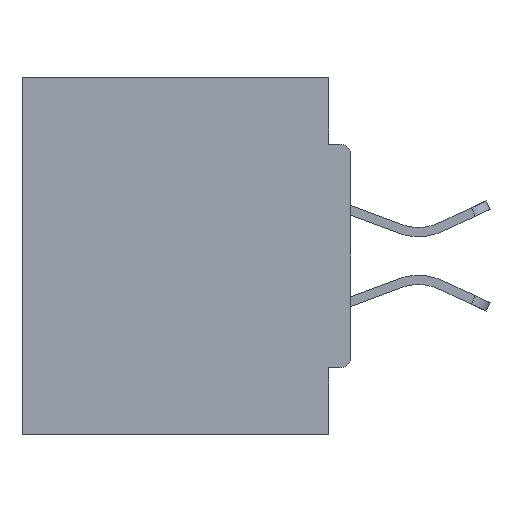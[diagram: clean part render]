
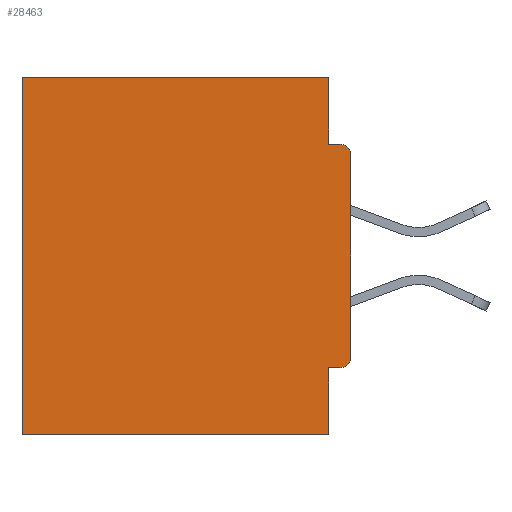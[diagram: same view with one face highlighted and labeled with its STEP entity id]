
A CAD part, left-side view. The second image highlights one B-rep face of the part: STEP entity #28463.
In plain terms, the highlighted planar face has unit normal (-1, 0, 0).
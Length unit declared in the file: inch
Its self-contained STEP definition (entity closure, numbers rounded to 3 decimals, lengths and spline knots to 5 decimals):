
#237 = CARTESIAN_POINT ( 'NONE',  ( 0.298, 0., -0.0935 ) ) ;
#345 = LINE ( 'NONE', #13694, #14508 ) ;
#370 = CARTESIAN_POINT ( 'NONE',  ( 0.298, 0.015, -0.4065 ) ) ;
#775 = CARTESIAN_POINT ( 'NONE',  ( 0.298, 0., 0. ) ) ;
#823 = CIRCLE ( 'NONE', #12966, 0.015 ) ;
#965 = CARTESIAN_POINT ( 'NONE',  ( 0.298, 0., -0.4065 ) ) ;
#1028 = EDGE_CURVE ( 'NONE', #24210, #27867, #21566, .T. ) ;
#1080 = DIRECTION ( 'NONE',  ( 0., 1., 0. ) ) ;
#1135 = DIRECTION ( 'NONE',  ( 0., 0., -1. ) ) ;
#2002 = CARTESIAN_POINT ( 'NONE',  ( 0.298, 0.46, -0.5 ) ) ;
#2322 = DIRECTION ( 'NONE',  ( 0., 0., -1. ) ) ;
#2392 = VECTOR ( 'NONE', #9474, 39.37008 ) ;
#2773 = VECTOR ( 'NONE', #23003, 39.37008 ) ;
#3357 = EDGE_CURVE ( 'NONE', #23537, #8832, #28068, .T. ) ;
#3462 = CARTESIAN_POINT ( 'NONE',  ( 0.298, 0.031, -0.4065 ) ) ;
#3472 = CARTESIAN_POINT ( 'NONE',  ( 0.298, 0., -0.1085 ) ) ;
#3827 = EDGE_CURVE ( 'NONE', #36233, #8108, #24027, .T. ) ;
#4195 = DIRECTION ( 'NONE',  ( 0., 1., 0. ) ) ;
#4475 = ORIENTED_EDGE ( 'NONE', *, *, #3827, .F. ) ;
#5060 = CARTESIAN_POINT ( 'NONE',  ( 0.298, 0.015, -0.0935 ) ) ;
#5098 = LINE ( 'NONE', #965, #11684 ) ;
#5111 = DIRECTION ( 'NONE',  ( -1., 0., 0. ) ) ;
#6636 = CARTESIAN_POINT ( 'NONE',  ( 0.298, 0.031, 0. ) ) ;
#7473 = LINE ( 'NONE', #20763, #22356 ) ;
#8108 = VERTEX_POINT ( 'NONE', #12264 ) ;
#8785 = ORIENTED_EDGE ( 'NONE', *, *, #11113, .F. ) ;
#8832 = VERTEX_POINT ( 'NONE', #5060 ) ;
#9336 = DIRECTION ( 'NONE',  ( 0., 0., -1. ) ) ;
#9474 = DIRECTION ( 'NONE',  ( 0., 0., -1. ) ) ;
#11113 = EDGE_CURVE ( 'NONE', #15037, #24613, #5098, .T. ) ;
#11594 = DIRECTION ( 'NONE',  ( 0., -1., 0. ) ) ;
#11684 = VECTOR ( 'NONE', #1080, 39.37008 ) ;
#12264 = CARTESIAN_POINT ( 'NONE',  ( 0.298, 0., -0.3915 ) ) ;
#12306 = AXIS2_PLACEMENT_3D ( 'NONE', #30603, #5111, #27496 ) ;
#12966 = AXIS2_PLACEMENT_3D ( 'NONE', #21600, #27003, #18953 ) ;
#13694 = CARTESIAN_POINT ( 'NONE',  ( 0.298, 0.031, -0.5 ) ) ;
#14508 = VECTOR ( 'NONE', #2322, 39.37008 ) ;
#14525 = CARTESIAN_POINT ( 'NONE',  ( 0.298, 0.031, -0.5 ) ) ;
#15037 = VERTEX_POINT ( 'NONE', #370 ) ;
#15137 = EDGE_LOOP ( 'NONE', ( #20660, #23714, #23108, #28283, #31960, #29684, #34054, #8785, #23698, #4475 ) ) ;
#15436 = CARTESIAN_POINT ( 'NONE',  ( 0.298, 0., -0.5 ) ) ;
#17260 = AXIS2_PLACEMENT_3D ( 'NONE', #775, #26269, #1135 ) ;
#17764 = CIRCLE ( 'NONE', #12306, 0.015 ) ;
#17913 = EDGE_CURVE ( 'NONE', #36233, #8832, #823, .T. ) ;
#18091 = PLANE ( 'NONE',  #17260 ) ;
#18953 = DIRECTION ( 'NONE',  ( 0., 0., -1. ) ) ;
#20490 = CARTESIAN_POINT ( 'NONE',  ( 0.298, 0.031, -0.0935 ) ) ;
#20660 = ORIENTED_EDGE ( 'NONE', *, *, #17913, .T. ) ;
#20763 = CARTESIAN_POINT ( 'NONE',  ( 0.298, 0.031, -0.5 ) ) ;
#20784 = CARTESIAN_POINT ( 'NONE',  ( 0.298, 0.46, 0. ) ) ;
#21309 = DIRECTION ( 'NONE',  ( 0., 1., 0. ) ) ;
#21566 = LINE ( 'NONE', #23907, #32193 ) ;
#21600 = CARTESIAN_POINT ( 'NONE',  ( 0.298, 0.015, -0.1085 ) ) ;
#22356 = VECTOR ( 'NONE', #9336, 39.37008 ) ;
#22581 = VECTOR ( 'NONE', #4195, 39.37008 ) ;
#23003 = DIRECTION ( 'NONE',  ( 0., 0., -1. ) ) ;
#23108 = ORIENTED_EDGE ( 'NONE', *, *, #26806, .F. ) ;
#23537 = VERTEX_POINT ( 'NONE', #20490 ) ;
#23698 = ORIENTED_EDGE ( 'NONE', *, *, #34289, .T. ) ;
#23714 = ORIENTED_EDGE ( 'NONE', *, *, #3357, .F. ) ;
#23907 = CARTESIAN_POINT ( 'NONE',  ( 0.298, 0., 0. ) ) ;
#24027 = LINE ( 'NONE', #27706, #2773 ) ;
#24210 = VERTEX_POINT ( 'NONE', #6636 ) ;
#24613 = VERTEX_POINT ( 'NONE', #3462 ) ;
#26269 = DIRECTION ( 'NONE',  ( 1., 0., 0. ) ) ;
#26775 = FACE_OUTER_BOUND ( 'NONE', #15137, .T. ) ;
#26806 = EDGE_CURVE ( 'NONE', #24210, #23537, #7473, .T. ) ;
#27003 = DIRECTION ( 'NONE',  ( -1., 0., 0. ) ) ;
#27466 = VERTEX_POINT ( 'NONE', #2002 ) ;
#27496 = DIRECTION ( 'NONE',  ( 0., 0., -1. ) ) ;
#27706 = CARTESIAN_POINT ( 'NONE',  ( 0.298, 0., 0. ) ) ;
#27867 = VERTEX_POINT ( 'NONE', #32192 ) ;
#28068 = LINE ( 'NONE', #237, #35184 ) ;
#28283 = ORIENTED_EDGE ( 'NONE', *, *, #1028, .T. ) ;
#28463 = ADVANCED_FACE ( 'NONE', ( #26775 ), #18091, .F. ) ;
#28839 = EDGE_CURVE ( 'NONE', #27867, #27466, #31206, .T. ) ;
#29684 = ORIENTED_EDGE ( 'NONE', *, *, #32641, .F. ) ;
#30067 = LINE ( 'NONE', #15436, #22581 ) ;
#30603 = CARTESIAN_POINT ( 'NONE',  ( 0.298, 0.015, -0.3915 ) ) ;
#31206 = LINE ( 'NONE', #20784, #2392 ) ;
#31960 = ORIENTED_EDGE ( 'NONE', *, *, #28839, .T. ) ;
#32192 = CARTESIAN_POINT ( 'NONE',  ( 0.298, 0.46, 0. ) ) ;
#32193 = VECTOR ( 'NONE', #21309, 39.37008 ) ;
#32641 = EDGE_CURVE ( 'NONE', #33796, #27466, #30067, .T. ) ;
#33796 = VERTEX_POINT ( 'NONE', #14525 ) ;
#34054 = ORIENTED_EDGE ( 'NONE', *, *, #36617, .F. ) ;
#34289 = EDGE_CURVE ( 'NONE', #15037, #8108, #17764, .T. ) ;
#35184 = VECTOR ( 'NONE', #11594, 39.37008 ) ;
#36233 = VERTEX_POINT ( 'NONE', #3472 ) ;
#36617 = EDGE_CURVE ( 'NONE', #24613, #33796, #345, .T. ) ;
